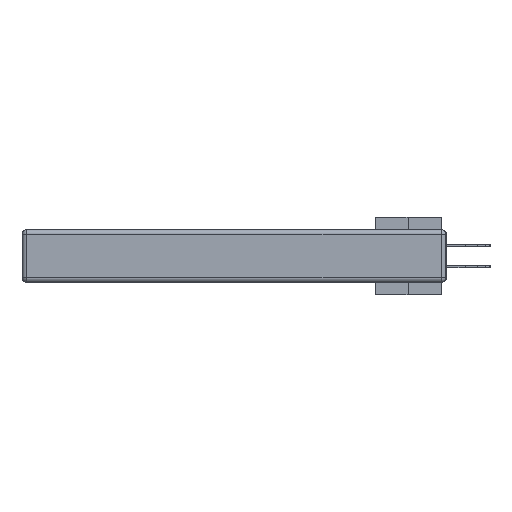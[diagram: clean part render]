
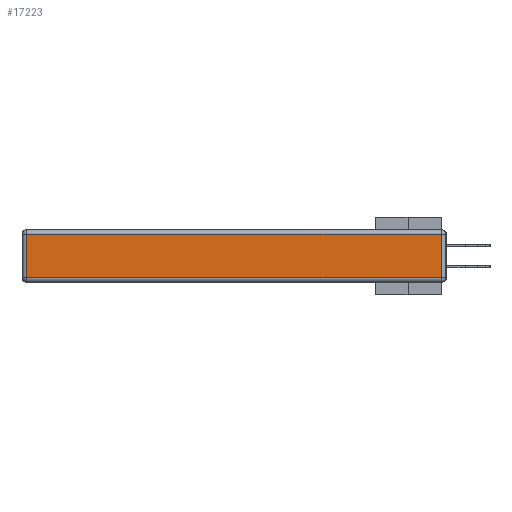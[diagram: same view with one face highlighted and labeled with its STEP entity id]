
A CAD part, left-side view. The second image highlights one B-rep face of the part: STEP entity #17223.
In plain terms, the highlighted planar face has unit normal (-1, 0, 0).
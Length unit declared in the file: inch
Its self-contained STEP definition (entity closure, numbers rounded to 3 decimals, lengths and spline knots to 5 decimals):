
#1055 = PLANE ( 'NONE',  #38443 ) ;
#1609 = LINE ( 'NONE', #25203, #42689 ) ;
#2012 = CARTESIAN_POINT ( 'NONE',  ( 0., 0.03, -0.313 ) ) ;
#2045 = VECTOR ( 'NONE', #40455, 39.37008 ) ;
#3327 = EDGE_CURVE ( 'NONE', #5511, #37468, #28284, .T. ) ;
#3561 = CARTESIAN_POINT ( 'NONE',  ( 0., 2.72, -0.03 ) ) ;
#4384 = DIRECTION ( 'NONE',  ( 0., 0., 1. ) ) ;
#4488 = CARTESIAN_POINT ( 'NONE',  ( 0., 2.72, -0.343 ) ) ;
#5511 = VERTEX_POINT ( 'NONE', #3561 ) ;
#6018 = ORIENTED_EDGE ( 'NONE', *, *, #8258, .T. ) ;
#6787 = ORIENTED_EDGE ( 'NONE', *, *, #27250, .T. ) ;
#8258 = EDGE_CURVE ( 'NONE', #10233, #14867, #1609, .T. ) ;
#10233 = VERTEX_POINT ( 'NONE', #2012 ) ;
#10537 = CARTESIAN_POINT ( 'NONE',  ( 0., 0.03, -0.03 ) ) ;
#11160 = CARTESIAN_POINT ( 'NONE',  ( 0., 0., -0.343 ) ) ;
#14259 = DIRECTION ( 'NONE',  ( 0., -1., 0. ) ) ;
#14867 = VERTEX_POINT ( 'NONE', #10537 ) ;
#15322 = ORIENTED_EDGE ( 'NONE', *, *, #3327, .T. ) ;
#17223 = ADVANCED_FACE ( 'NONE', ( #26101 ), #1055, .T. ) ;
#19025 = VECTOR ( 'NONE', #39118, 39.37008 ) ;
#20604 = VECTOR ( 'NONE', #14259, 39.37008 ) ;
#25056 = DIRECTION ( 'NONE',  ( -1., 0., 0. ) ) ;
#25203 = CARTESIAN_POINT ( 'NONE',  ( 0., 0.03, -0.343 ) ) ;
#26101 = FACE_OUTER_BOUND ( 'NONE', #27685, .T. ) ;
#27250 = EDGE_CURVE ( 'NONE', #37468, #10233, #29912, .T. ) ;
#27685 = EDGE_LOOP ( 'NONE', ( #6787, #6018, #28987, #15322 ) ) ;
#28284 = LINE ( 'NONE', #4488, #19025 ) ;
#28607 = CARTESIAN_POINT ( 'NONE',  ( 0., 0., -0.313 ) ) ;
#28987 = ORIENTED_EDGE ( 'NONE', *, *, #29680, .T. ) ;
#29680 = EDGE_CURVE ( 'NONE', #14867, #5511, #40409, .T. ) ;
#29912 = LINE ( 'NONE', #28607, #20604 ) ;
#31784 = DIRECTION ( 'NONE',  ( 0., 0., 1. ) ) ;
#36174 = CARTESIAN_POINT ( 'NONE',  ( 0., 2.72, -0.313 ) ) ;
#36927 = CARTESIAN_POINT ( 'NONE',  ( 0., 2.75, -0.03 ) ) ;
#37468 = VERTEX_POINT ( 'NONE', #36174 ) ;
#38443 = AXIS2_PLACEMENT_3D ( 'NONE', #11160, #25056, #4384 ) ;
#39118 = DIRECTION ( 'NONE',  ( 0., 0., -1. ) ) ;
#40409 = LINE ( 'NONE', #36927, #2045 ) ;
#40455 = DIRECTION ( 'NONE',  ( 0., 1., 0. ) ) ;
#42689 = VECTOR ( 'NONE', #31784, 39.37008 ) ;
